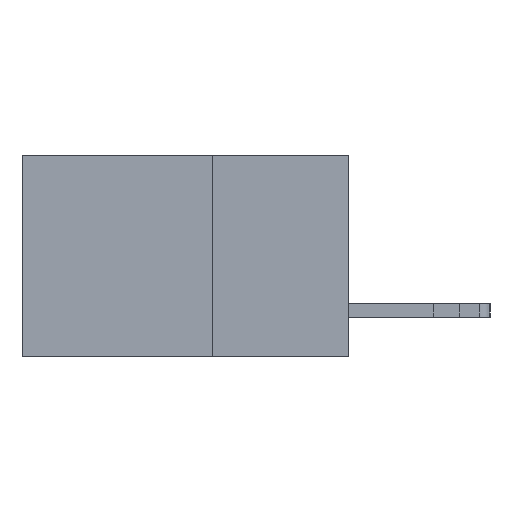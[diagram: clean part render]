
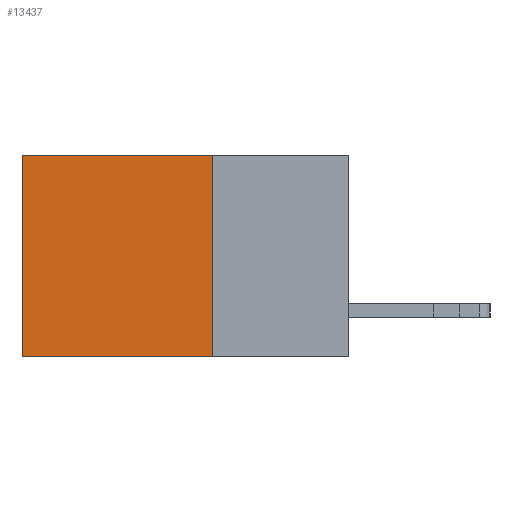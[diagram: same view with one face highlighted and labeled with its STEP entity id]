
A CAD part, left-side view. The second image highlights one B-rep face of the part: STEP entity #13437.
In plain terms, the highlighted planar face has unit normal (-1, 0, 0).
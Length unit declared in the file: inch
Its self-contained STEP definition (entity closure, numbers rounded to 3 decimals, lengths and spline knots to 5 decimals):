
#219 = DIRECTION ( 'NONE',  ( 0., 0., -1. ) ) ;
#293 = LINE ( 'NONE', #8758, #18135 ) ;
#2698 = VERTEX_POINT ( 'NONE', #4508 ) ;
#2949 = DIRECTION ( 'NONE',  ( 0., 0., -1. ) ) ;
#4508 = CARTESIAN_POINT ( 'NONE',  ( 0.298, 0.25, -0.37 ) ) ;
#4934 = EDGE_LOOP ( 'NONE', ( #6764, #16939, #14328, #17279 ) ) ;
#5558 = LINE ( 'NONE', #17034, #12639 ) ;
#6764 = ORIENTED_EDGE ( 'NONE', *, *, #15843, .T. ) ;
#7137 = VECTOR ( 'NONE', #14395, 39.37008 ) ;
#7188 = PLANE ( 'NONE',  #16391 ) ;
#8054 = CARTESIAN_POINT ( 'NONE',  ( 0.298, 0.25, -0.37 ) ) ;
#8715 = VERTEX_POINT ( 'NONE', #14769 ) ;
#8758 = CARTESIAN_POINT ( 'NONE',  ( 0.298, 0.6, 0. ) ) ;
#9046 = VERTEX_POINT ( 'NONE', #12676 ) ;
#10120 = DIRECTION ( 'NONE',  ( 0., 0., -1. ) ) ;
#10258 = EDGE_CURVE ( 'NONE', #13069, #8715, #18007, .T. ) ;
#11422 = DIRECTION ( 'NONE',  ( 1., 0., 0. ) ) ;
#12639 = VECTOR ( 'NONE', #10120, 39.37008 ) ;
#12676 = CARTESIAN_POINT ( 'NONE',  ( 0.298, 0.6, -0.37 ) ) ;
#12796 = CARTESIAN_POINT ( 'NONE',  ( 0.298, 0.25, 0. ) ) ;
#13018 = CARTESIAN_POINT ( 'NONE',  ( 0.298, 0.25, 0. ) ) ;
#13069 = VERTEX_POINT ( 'NONE', #15933 ) ;
#13437 = ADVANCED_FACE ( 'NONE', ( #15773 ), #7188, .F. ) ;
#13574 = LINE ( 'NONE', #8054, #15954 ) ;
#14328 = ORIENTED_EDGE ( 'NONE', *, *, #17960, .F. ) ;
#14395 = DIRECTION ( 'NONE',  ( 0., 1., 0. ) ) ;
#14769 = CARTESIAN_POINT ( 'NONE',  ( 0.298, 0.6, 0. ) ) ;
#15171 = DIRECTION ( 'NONE',  ( 0., 1., 0. ) ) ;
#15773 = FACE_OUTER_BOUND ( 'NONE', #4934, .T. ) ;
#15843 = EDGE_CURVE ( 'NONE', #8715, #9046, #293, .T. ) ;
#15933 = CARTESIAN_POINT ( 'NONE',  ( 0.298, 0.25, 0. ) ) ;
#15954 = VECTOR ( 'NONE', #15171, 39.37008 ) ;
#16391 = AXIS2_PLACEMENT_3D ( 'NONE', #12796, #11422, #2949 ) ;
#16939 = ORIENTED_EDGE ( 'NONE', *, *, #17152, .F. ) ;
#17034 = CARTESIAN_POINT ( 'NONE',  ( 0.298, 0.25, 0. ) ) ;
#17152 = EDGE_CURVE ( 'NONE', #2698, #9046, #13574, .T. ) ;
#17279 = ORIENTED_EDGE ( 'NONE', *, *, #10258, .T. ) ;
#17960 = EDGE_CURVE ( 'NONE', #13069, #2698, #5558, .T. ) ;
#18007 = LINE ( 'NONE', #13018, #7137 ) ;
#18135 = VECTOR ( 'NONE', #219, 39.37008 ) ;
